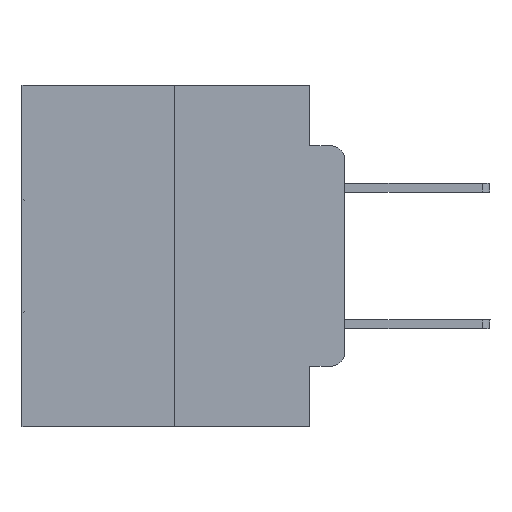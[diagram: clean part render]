
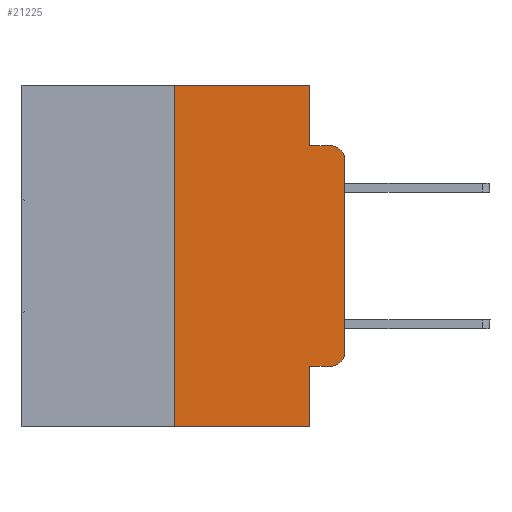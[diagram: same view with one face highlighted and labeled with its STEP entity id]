
A CAD part, left-side view. The second image highlights one B-rep face of the part: STEP entity #21225.
In plain terms, the highlighted planar face has unit normal (-1, 0, 0).
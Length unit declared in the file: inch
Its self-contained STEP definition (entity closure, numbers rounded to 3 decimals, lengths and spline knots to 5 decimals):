
#461 = VECTOR ( 'NONE', #11924, 39.37008 ) ;
#695 = AXIS2_PLACEMENT_3D ( 'NONE', #1628, #1831, #29979 ) ;
#777 = VERTEX_POINT ( 'NONE', #9263 ) ;
#1496 = DIRECTION ( 'NONE',  ( -1., 0., 0. ) ) ;
#1551 = LINE ( 'NONE', #28513, #461 ) ;
#1628 = CARTESIAN_POINT ( 'NONE',  ( 0., 0.02, -0.1085 ) ) ;
#1831 = DIRECTION ( 'NONE',  ( -1., 0., 0. ) ) ;
#1957 = CIRCLE ( 'NONE', #695, 0.02 ) ;
#2778 = ORIENTED_EDGE ( 'NONE', *, *, #23406, .T. ) ;
#3242 = ORIENTED_EDGE ( 'NONE', *, *, #29717, .F. ) ;
#3842 = CARTESIAN_POINT ( 'NONE',  ( 0., 0.051, -0.5 ) ) ;
#4009 = CARTESIAN_POINT ( 'NONE',  ( 0., 0., -0.1085 ) ) ;
#4161 = LINE ( 'NONE', #23742, #9282 ) ;
#4461 = VECTOR ( 'NONE', #4799, 39.37008 ) ;
#4497 = ORIENTED_EDGE ( 'NONE', *, *, #20495, .T. ) ;
#4799 = DIRECTION ( 'NONE',  ( 0., 0., 1. ) ) ;
#5558 = EDGE_CURVE ( 'NONE', #777, #21962, #15488, .T. ) ;
#5562 = EDGE_CURVE ( 'NONE', #23090, #11097, #22867, .T. ) ;
#5637 = CARTESIAN_POINT ( 'NONE',  ( 0., 0.473, 0. ) ) ;
#5873 = AXIS2_PLACEMENT_3D ( 'NONE', #27215, #1496, #6359 ) ;
#6322 = VECTOR ( 'NONE', #22284, 39.37008 ) ;
#6359 = DIRECTION ( 'NONE',  ( 0., 0., -1. ) ) ;
#6993 = FACE_OUTER_BOUND ( 'NONE', #22694, .T. ) ;
#7079 = EDGE_CURVE ( 'NONE', #21962, #23090, #11364, .T. ) ;
#7560 = ORIENTED_EDGE ( 'NONE', *, *, #5562, .F. ) ;
#7574 = DIRECTION ( 'NONE',  ( 0., 0., 1. ) ) ;
#8177 = CARTESIAN_POINT ( 'NONE',  ( 0., 0., -0.3915 ) ) ;
#9263 = CARTESIAN_POINT ( 'NONE',  ( 0., 0.25, 0. ) ) ;
#9282 = VECTOR ( 'NONE', #7574, 39.37008 ) ;
#9514 = CARTESIAN_POINT ( 'NONE',  ( 0., 0.051, -0.0885 ) ) ;
#9773 = AXIS2_PLACEMENT_3D ( 'NONE', #25705, #11766, #18775 ) ;
#10572 = EDGE_CURVE ( 'NONE', #30191, #28803, #13736, .T. ) ;
#11097 = VERTEX_POINT ( 'NONE', #27029 ) ;
#11289 = ORIENTED_EDGE ( 'NONE', *, *, #20394, .T. ) ;
#11364 = LINE ( 'NONE', #23462, #21664 ) ;
#11766 = DIRECTION ( 'NONE',  ( 1., 0., 0. ) ) ;
#11853 = CARTESIAN_POINT ( 'NONE',  ( 0., 0., 0. ) ) ;
#11924 = DIRECTION ( 'NONE',  ( 0., -1., 0. ) ) ;
#13736 = LINE ( 'NONE', #26966, #14471 ) ;
#14015 = VECTOR ( 'NONE', #17226, 39.37008 ) ;
#14471 = VECTOR ( 'NONE', #29311, 39.37008 ) ;
#15488 = LINE ( 'NONE', #5637, #14015 ) ;
#15918 = CARTESIAN_POINT ( 'NONE',  ( 0., 0.02, -0.4115 ) ) ;
#16598 = PLANE ( 'NONE',  #9773 ) ;
#16820 = ORIENTED_EDGE ( 'NONE', *, *, #7079, .F. ) ;
#17226 = DIRECTION ( 'NONE',  ( 0., -1., 0. ) ) ;
#17494 = ORIENTED_EDGE ( 'NONE', *, *, #10572, .F. ) ;
#18603 = DIRECTION ( 'NONE',  ( 0., 0., -1. ) ) ;
#18619 = VERTEX_POINT ( 'NONE', #21219 ) ;
#18775 = DIRECTION ( 'NONE',  ( 0., 0., -1. ) ) ;
#19820 = ORIENTED_EDGE ( 'NONE', *, *, #5558, .F. ) ;
#19902 = LINE ( 'NONE', #21535, #22479 ) ;
#20394 = EDGE_CURVE ( 'NONE', #21602, #26647, #24722, .T. ) ;
#20495 = EDGE_CURVE ( 'NONE', #18619, #28803, #19902, .T. ) ;
#21219 = CARTESIAN_POINT ( 'NONE',  ( 0., 0.25, -0.5 ) ) ;
#21225 = ADVANCED_FACE ( 'NONE', ( #6993 ), #16598, .F. ) ;
#21535 = CARTESIAN_POINT ( 'NONE',  ( 0., 0.473, -0.5 ) ) ;
#21602 = VERTEX_POINT ( 'NONE', #8177 ) ;
#21664 = VECTOR ( 'NONE', #18603, 39.37008 ) ;
#21962 = VERTEX_POINT ( 'NONE', #28422 ) ;
#22284 = DIRECTION ( 'NONE',  ( 0., -1., 0. ) ) ;
#22479 = VECTOR ( 'NONE', #26077, 39.37008 ) ;
#22694 = EDGE_LOOP ( 'NONE', ( #11289, #23373, #7560, #16820, #19820, #3242, #4497, #17494, #23335, #2778 ) ) ;
#22867 = LINE ( 'NONE', #29362, #6322 ) ;
#23090 = VERTEX_POINT ( 'NONE', #9514 ) ;
#23335 = ORIENTED_EDGE ( 'NONE', *, *, #30338, .T. ) ;
#23373 = ORIENTED_EDGE ( 'NONE', *, *, #29481, .T. ) ;
#23406 = EDGE_CURVE ( 'NONE', #26145, #21602, #24202, .T. ) ;
#23462 = CARTESIAN_POINT ( 'NONE',  ( 0., 0.051, 0. ) ) ;
#23742 = CARTESIAN_POINT ( 'NONE',  ( 0., 0.25, 0. ) ) ;
#24202 = CIRCLE ( 'NONE', #5873, 0.02 ) ;
#24722 = LINE ( 'NONE', #11853, #4461 ) ;
#25705 = CARTESIAN_POINT ( 'NONE',  ( 0., 0.473, 0. ) ) ;
#25752 = CARTESIAN_POINT ( 'NONE',  ( 0., 0.051, -0.4115 ) ) ;
#26077 = DIRECTION ( 'NONE',  ( 0., -1., 0. ) ) ;
#26145 = VERTEX_POINT ( 'NONE', #15918 ) ;
#26647 = VERTEX_POINT ( 'NONE', #4009 ) ;
#26966 = CARTESIAN_POINT ( 'NONE',  ( 0., 0.051, 0. ) ) ;
#27029 = CARTESIAN_POINT ( 'NONE',  ( 0., 0.02, -0.0885 ) ) ;
#27215 = CARTESIAN_POINT ( 'NONE',  ( 0., 0.02, -0.3915 ) ) ;
#28422 = CARTESIAN_POINT ( 'NONE',  ( 0., 0.051, 0. ) ) ;
#28513 = CARTESIAN_POINT ( 'NONE',  ( 0., 0.051, -0.4115 ) ) ;
#28803 = VERTEX_POINT ( 'NONE', #3842 ) ;
#29311 = DIRECTION ( 'NONE',  ( 0., 0., -1. ) ) ;
#29362 = CARTESIAN_POINT ( 'NONE',  ( 0., 0.051, -0.0885 ) ) ;
#29481 = EDGE_CURVE ( 'NONE', #26647, #11097, #1957, .T. ) ;
#29717 = EDGE_CURVE ( 'NONE', #18619, #777, #4161, .T. ) ;
#29979 = DIRECTION ( 'NONE',  ( 0., 0., -1. ) ) ;
#30191 = VERTEX_POINT ( 'NONE', #25752 ) ;
#30338 = EDGE_CURVE ( 'NONE', #30191, #26145, #1551, .T. ) ;
